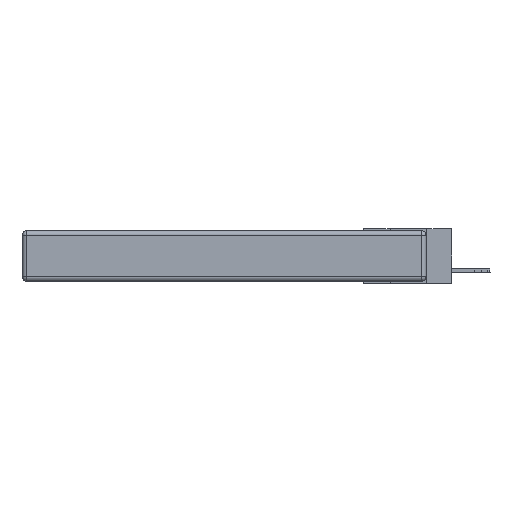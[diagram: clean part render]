
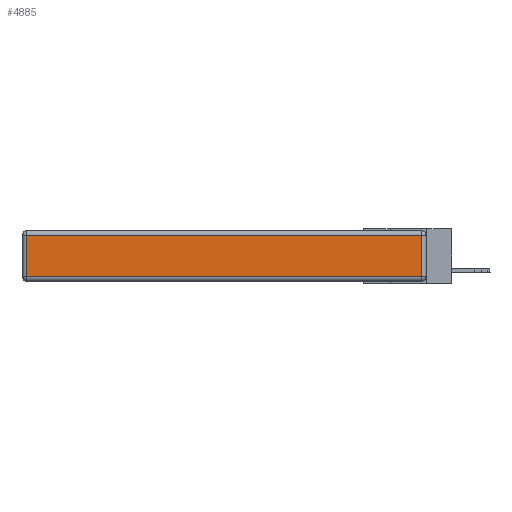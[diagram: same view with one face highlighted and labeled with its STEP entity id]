
A CAD part, left-side view. The second image highlights one B-rep face of the part: STEP entity #4885.
In plain terms, the highlighted planar face has unit normal (-1, 0, 0).
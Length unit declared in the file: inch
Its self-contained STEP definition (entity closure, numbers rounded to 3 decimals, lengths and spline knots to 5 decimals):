
#603 = CARTESIAN_POINT ( 'NONE',  ( 0., 2.75, -0.03 ) ) ;
#1127 = LINE ( 'NONE', #3329, #20410 ) ;
#1229 = VERTEX_POINT ( 'NONE', #5345 ) ;
#1293 = EDGE_CURVE ( 'NONE', #18067, #1229, #1127, .T. ) ;
#1394 = EDGE_LOOP ( 'NONE', ( #9153, #3796, #2119, #3117 ) ) ;
#2119 = ORIENTED_EDGE ( 'NONE', *, *, #14281, .T. ) ;
#3117 = ORIENTED_EDGE ( 'NONE', *, *, #1293, .T. ) ;
#3329 = CARTESIAN_POINT ( 'NONE',  ( 0., 2.72, -0.343 ) ) ;
#3796 = ORIENTED_EDGE ( 'NONE', *, *, #21870, .T. ) ;
#4513 = CARTESIAN_POINT ( 'NONE',  ( 0., 0.03, -0.343 ) ) ;
#4885 = ADVANCED_FACE ( 'NONE', ( #6355 ), #16145, .T. ) ;
#5345 = CARTESIAN_POINT ( 'NONE',  ( 0., 2.72, -0.313 ) ) ;
#5385 = EDGE_CURVE ( 'NONE', #1229, #20723, #20340, .T. ) ;
#6081 = DIRECTION ( 'NONE',  ( 0., 0., 1. ) ) ;
#6355 = FACE_OUTER_BOUND ( 'NONE', #1394, .T. ) ;
#7083 = DIRECTION ( 'NONE',  ( 0., 0., -1. ) ) ;
#7193 = VECTOR ( 'NONE', #15716, 39.37008 ) ;
#8814 = CARTESIAN_POINT ( 'NONE',  ( 0., 2.72, -0.03 ) ) ;
#9153 = ORIENTED_EDGE ( 'NONE', *, *, #5385, .T. ) ;
#9181 = VECTOR ( 'NONE', #11954, 39.37008 ) ;
#11910 = DIRECTION ( 'NONE',  ( -1., 0., 0. ) ) ;
#11954 = DIRECTION ( 'NONE',  ( 0., 1., 0. ) ) ;
#13330 = AXIS2_PLACEMENT_3D ( 'NONE', #23101, #11910, #14359 ) ;
#14185 = LINE ( 'NONE', #603, #9181 ) ;
#14281 = EDGE_CURVE ( 'NONE', #21141, #18067, #14185, .T. ) ;
#14359 = DIRECTION ( 'NONE',  ( 0., 0., 1. ) ) ;
#15019 = CARTESIAN_POINT ( 'NONE',  ( 0., 0.03, -0.313 ) ) ;
#15716 = DIRECTION ( 'NONE',  ( 0., -1., 0. ) ) ;
#16145 = PLANE ( 'NONE',  #13330 ) ;
#17431 = LINE ( 'NONE', #4513, #18883 ) ;
#17818 = CARTESIAN_POINT ( 'NONE',  ( 0., 0., -0.313 ) ) ;
#18067 = VERTEX_POINT ( 'NONE', #8814 ) ;
#18883 = VECTOR ( 'NONE', #6081, 39.37008 ) ;
#20340 = LINE ( 'NONE', #17818, #7193 ) ;
#20410 = VECTOR ( 'NONE', #7083, 39.37008 ) ;
#20723 = VERTEX_POINT ( 'NONE', #15019 ) ;
#21141 = VERTEX_POINT ( 'NONE', #22259 ) ;
#21870 = EDGE_CURVE ( 'NONE', #20723, #21141, #17431, .T. ) ;
#22259 = CARTESIAN_POINT ( 'NONE',  ( 0., 0.03, -0.03 ) ) ;
#23101 = CARTESIAN_POINT ( 'NONE',  ( 0., 0., -0.343 ) ) ;
